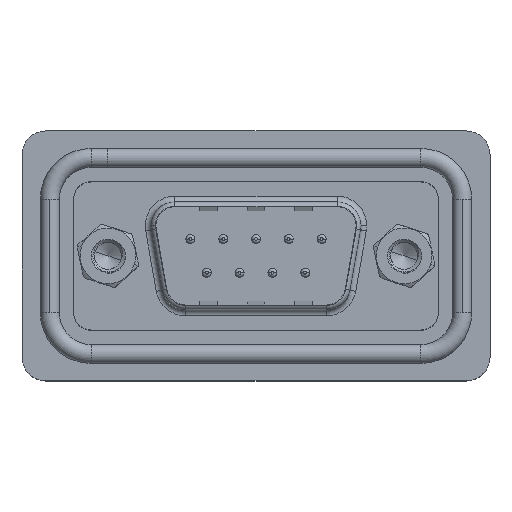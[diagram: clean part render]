
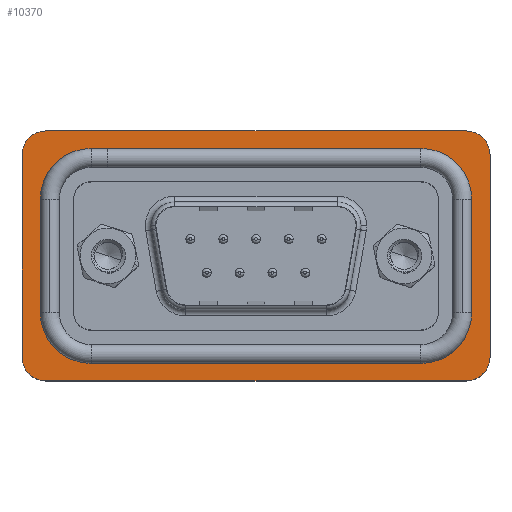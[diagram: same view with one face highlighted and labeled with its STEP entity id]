
A CAD part, top view. The second image highlights one B-rep face of the part: STEP entity #10370.
In plain terms, the highlighted planar face has unit normal (0, 0, 1).
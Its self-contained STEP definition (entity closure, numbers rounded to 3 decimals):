
#96 = LINE ( 'NONE', #14148, #6378 ) ;
#99 = DIRECTION ( 'NONE',  ( 0., 0., 1. ) ) ;
#540 = CIRCLE ( 'NONE', #13585, 4.3 ) ;
#606 = EDGE_CURVE ( 'NONE', #3414, #6151, #19658, .T. ) ;
#797 = CARTESIAN_POINT ( 'NONE',  ( 30.705, -4.775, 0.5 ) ) ;
#854 = VERTEX_POINT ( 'NONE', #5280 ) ;
#891 = CARTESIAN_POINT ( 'NONE',  ( 26.405, 9.075, 0.5 ) ) ;
#929 = VECTOR ( 'NONE', #9782, 1000. ) ;
#997 = CARTESIAN_POINT ( 'NONE',  ( 26.405, 4.775, 0.5 ) ) ;
#1078 = ORIENTED_EDGE ( 'NONE', *, *, #3339, .F. ) ;
#1106 = CARTESIAN_POINT ( 'NONE',  ( -7.25, -8.55, 0.5 ) ) ;
#1278 = VECTOR ( 'NONE', #11512, 1000. ) ;
#1297 = ORIENTED_EDGE ( 'NONE', *, *, #1497, .T. ) ;
#1317 = VERTEX_POINT ( 'NONE', #15199 ) ;
#1422 = ORIENTED_EDGE ( 'NONE', *, *, #11343, .F. ) ;
#1497 = EDGE_CURVE ( 'NONE', #4690, #17657, #9756, .T. ) ;
#1758 = DIRECTION ( 'NONE',  ( 0., 0., 1. ) ) ;
#1893 = VERTEX_POINT ( 'NONE', #797 ) ;
#1958 = DIRECTION ( 'NONE',  ( 1., 0., 0. ) ) ;
#2152 = LINE ( 'NONE', #5312, #1278 ) ;
#2167 = CARTESIAN_POINT ( 'NONE',  ( 30.705, -4.775, 0.5 ) ) ;
#2875 = CARTESIAN_POINT ( 'NONE',  ( 30.25, 8.55, 0.5 ) ) ;
#2889 = DIRECTION ( 'NONE',  ( 0., 0., 1. ) ) ;
#3090 = DIRECTION ( 'NONE',  ( 1., 0., 0. ) ) ;
#3299 = DIRECTION ( 'NONE',  ( 1., 0., 0. ) ) ;
#3339 = EDGE_CURVE ( 'NONE', #8098, #14010, #8241, .T. ) ;
#3414 = VERTEX_POINT ( 'NONE', #17522 ) ;
#3664 = CARTESIAN_POINT ( 'NONE',  ( -7.25, 8.55, 0.5 ) ) ;
#4052 = ORIENTED_EDGE ( 'NONE', *, *, #11380, .F. ) ;
#4205 = CARTESIAN_POINT ( 'NONE',  ( 30.705, 4.775, 0.5 ) ) ;
#4254 = AXIS2_PLACEMENT_3D ( 'NONE', #13463, #19673, #5709 ) ;
#4343 = ORIENTED_EDGE ( 'NONE', *, *, #19286, .T. ) ;
#4385 = ORIENTED_EDGE ( 'NONE', *, *, #15082, .T. ) ;
#4536 = VERTEX_POINT ( 'NONE', #15399 ) ;
#4690 = VERTEX_POINT ( 'NONE', #15882 ) ;
#4802 = VECTOR ( 'NONE', #7313, 1000. ) ;
#4869 = CARTESIAN_POINT ( 'NONE',  ( -5.25, -10.55, 0.5 ) ) ;
#5123 = LINE ( 'NONE', #2167, #19468 ) ;
#5236 = AXIS2_PLACEMENT_3D ( 'NONE', #19566, #7020, #11823 ) ;
#5280 = CARTESIAN_POINT ( 'NONE',  ( 30.25, 10.55, 0.5 ) ) ;
#5312 = CARTESIAN_POINT ( 'NONE',  ( -1.405, -9.075, 0.5 ) ) ;
#5325 = AXIS2_PLACEMENT_3D ( 'NONE', #14061, #99, #1958 ) ;
#5561 = ORIENTED_EDGE ( 'NONE', *, *, #20165, .T. ) ;
#5697 = DIRECTION ( 'NONE',  ( 0., 0., 1. ) ) ;
#5709 = DIRECTION ( 'NONE',  ( 1., 0., 0. ) ) ;
#5882 = AXIS2_PLACEMENT_3D ( 'NONE', #9493, #1758, #3090 ) ;
#5897 = VECTOR ( 'NONE', #3299, 1000. ) ;
#5939 = DIRECTION ( 'NONE',  ( -1., 0., 0. ) ) ;
#6151 = VERTEX_POINT ( 'NONE', #3664 ) ;
#6205 = DIRECTION ( 'NONE',  ( 0., 0., 1. ) ) ;
#6314 = DIRECTION ( 'NONE',  ( 0., 1., 0. ) ) ;
#6378 = VECTOR ( 'NONE', #6314, 1000. ) ;
#6390 = EDGE_CURVE ( 'NONE', #16327, #7993, #9828, .T. ) ;
#6750 = ORIENTED_EDGE ( 'NONE', *, *, #12729, .T. ) ;
#7020 = DIRECTION ( 'NONE',  ( 0., 0., 1. ) ) ;
#7208 = DIRECTION ( 'NONE',  ( 1., 0., 0. ) ) ;
#7313 = DIRECTION ( 'NONE',  ( 0., -1., 0. ) ) ;
#7444 = PLANE ( 'NONE',  #19441 ) ;
#7993 = VERTEX_POINT ( 'NONE', #10981 ) ;
#8098 = VERTEX_POINT ( 'NONE', #18004 ) ;
#8110 = EDGE_CURVE ( 'NONE', #1317, #8098, #17588, .T. ) ;
#8124 = DIRECTION ( 'NONE',  ( 1., 0., 0. ) ) ;
#8241 = CIRCLE ( 'NONE', #5325, 4.3 ) ;
#8303 = CIRCLE ( 'NONE', #10910, 2. ) ;
#8442 = ORIENTED_EDGE ( 'NONE', *, *, #12794, .F. ) ;
#8841 = LINE ( 'NONE', #13536, #17187 ) ;
#8902 = EDGE_LOOP ( 'NONE', ( #4052, #18088, #14301, #8442, #16794, #1422, #1078, #11259 ) ) ;
#8923 = AXIS2_PLACEMENT_3D ( 'NONE', #18648, #6205, #8124 ) ;
#8973 = FACE_OUTER_BOUND ( 'NONE', #13426, .T. ) ;
#8990 = CARTESIAN_POINT ( 'NONE',  ( -5.705, 4.775, 0.5 ) ) ;
#9073 = DIRECTION ( 'NONE',  ( 1., 0., 0. ) ) ;
#9283 = CARTESIAN_POINT ( 'NONE',  ( -5.25, -8.55, 0.5 ) ) ;
#9493 = CARTESIAN_POINT ( 'NONE',  ( 30.25, -8.55, 0.5 ) ) ;
#9601 = DIRECTION ( 'NONE',  ( 0., 1., 0. ) ) ;
#9606 = CARTESIAN_POINT ( 'NONE',  ( -5.705, -4.775, 0.5 ) ) ;
#9682 = CARTESIAN_POINT ( 'NONE',  ( 30.25, 10.55, 0.5 ) ) ;
#9756 = CIRCLE ( 'NONE', #5882, 2. ) ;
#9774 = VERTEX_POINT ( 'NONE', #4869 ) ;
#9782 = DIRECTION ( 'NONE',  ( -1., 0., 0. ) ) ;
#9828 = CIRCLE ( 'NONE', #16680, 4.3 ) ;
#9946 = DIRECTION ( 'NONE',  ( -1., 0., 0. ) ) ;
#10351 = LINE ( 'NONE', #1106, #4802 ) ;
#10370 = ADVANCED_FACE ( 'NONE', ( #15583, #8973 ), #7444, .T. ) ;
#10432 = VECTOR ( 'NONE', #9946, 1000. ) ;
#10876 = VERTEX_POINT ( 'NONE', #14782 ) ;
#10910 = AXIS2_PLACEMENT_3D ( 'NONE', #9283, #2889, #5939 ) ;
#10981 = CARTESIAN_POINT ( 'NONE',  ( -1.405, -9.075, 0.5 ) ) ;
#11259 = ORIENTED_EDGE ( 'NONE', *, *, #8110, .F. ) ;
#11343 = EDGE_CURVE ( 'NONE', #14010, #16327, #8841, .T. ) ;
#11380 = EDGE_CURVE ( 'NONE', #16590, #1317, #540, .T. ) ;
#11383 = EDGE_CURVE ( 'NONE', #6151, #4536, #10351, .T. ) ;
#11512 = DIRECTION ( 'NONE',  ( 1., 0., 0. ) ) ;
#11823 = DIRECTION ( 'NONE',  ( 1., 0., 0. ) ) ;
#11830 = CARTESIAN_POINT ( 'NONE',  ( 32.25, -8.55, 0.5 ) ) ;
#11968 = ORIENTED_EDGE ( 'NONE', *, *, #606, .T. ) ;
#11974 = ORIENTED_EDGE ( 'NONE', *, *, #17279, .T. ) ;
#12003 = DIRECTION ( 'NONE',  ( 0., -1., 0. ) ) ;
#12668 = CARTESIAN_POINT ( 'NONE',  ( 30.25, -10.55, 0.5 ) ) ;
#12729 = EDGE_CURVE ( 'NONE', #854, #3414, #12853, .T. ) ;
#12794 = EDGE_CURVE ( 'NONE', #7993, #10876, #2152, .T. ) ;
#12853 = LINE ( 'NONE', #9682, #929 ) ;
#12856 = EDGE_CURVE ( 'NONE', #1893, #16590, #5123, .T. ) ;
#13426 = EDGE_LOOP ( 'NONE', ( #4385, #6750, #11968, #14557, #4343, #11974, #1297, #5561 ) ) ;
#13463 = CARTESIAN_POINT ( 'NONE',  ( 26.405, -4.775, 0.5 ) ) ;
#13536 = CARTESIAN_POINT ( 'NONE',  ( -5.705, 4.775, 0.5 ) ) ;
#13549 = CARTESIAN_POINT ( 'NONE',  ( -1.405, -4.775, 0.5 ) ) ;
#13585 = AXIS2_PLACEMENT_3D ( 'NONE', #997, #15048, #7208 ) ;
#14010 = VERTEX_POINT ( 'NONE', #8990 ) ;
#14061 = CARTESIAN_POINT ( 'NONE',  ( -1.405, 4.775, 0.5 ) ) ;
#14148 = CARTESIAN_POINT ( 'NONE',  ( 32.25, -8.55, 0.5 ) ) ;
#14301 = ORIENTED_EDGE ( 'NONE', *, *, #14434, .F. ) ;
#14434 = EDGE_CURVE ( 'NONE', #10876, #1893, #15945, .T. ) ;
#14557 = ORIENTED_EDGE ( 'NONE', *, *, #11383, .T. ) ;
#14782 = CARTESIAN_POINT ( 'NONE',  ( 26.405, -9.075, 0.5 ) ) ;
#15048 = DIRECTION ( 'NONE',  ( 0., 0., 1. ) ) ;
#15082 = EDGE_CURVE ( 'NONE', #19301, #854, #18580, .T. ) ;
#15199 = CARTESIAN_POINT ( 'NONE',  ( 26.405, 9.075, 0.5 ) ) ;
#15399 = CARTESIAN_POINT ( 'NONE',  ( -7.25, -8.55, 0.5 ) ) ;
#15583 = FACE_BOUND ( 'NONE', #8902, .T. ) ;
#15882 = CARTESIAN_POINT ( 'NONE',  ( 30.25, -10.55, 0.5 ) ) ;
#15945 = CIRCLE ( 'NONE', #4254, 4.3 ) ;
#16327 = VERTEX_POINT ( 'NONE', #9606 ) ;
#16590 = VERTEX_POINT ( 'NONE', #4205 ) ;
#16680 = AXIS2_PLACEMENT_3D ( 'NONE', #13549, #5697, #19764 ) ;
#16794 = ORIENTED_EDGE ( 'NONE', *, *, #6390, .F. ) ;
#17187 = VECTOR ( 'NONE', #12003, 1000. ) ;
#17235 = LINE ( 'NONE', #12668, #5897 ) ;
#17279 = EDGE_CURVE ( 'NONE', #9774, #4690, #17235, .T. ) ;
#17522 = CARTESIAN_POINT ( 'NONE',  ( -5.25, 10.55, 0.5 ) ) ;
#17588 = LINE ( 'NONE', #891, #10432 ) ;
#17657 = VERTEX_POINT ( 'NONE', #11830 ) ;
#18004 = CARTESIAN_POINT ( 'NONE',  ( -1.405, 9.075, 0.5 ) ) ;
#18088 = ORIENTED_EDGE ( 'NONE', *, *, #12856, .F. ) ;
#18580 = CIRCLE ( 'NONE', #5236, 2. ) ;
#18648 = CARTESIAN_POINT ( 'NONE',  ( -5.25, 8.55, 0.5 ) ) ;
#19286 = EDGE_CURVE ( 'NONE', #4536, #9774, #8303, .T. ) ;
#19301 = VERTEX_POINT ( 'NONE', #19797 ) ;
#19441 = AXIS2_PLACEMENT_3D ( 'NONE', #2875, #19890, #9073 ) ;
#19468 = VECTOR ( 'NONE', #9601, 1000. ) ;
#19566 = CARTESIAN_POINT ( 'NONE',  ( 30.25, 8.55, 0.5 ) ) ;
#19658 = CIRCLE ( 'NONE', #8923, 2. ) ;
#19673 = DIRECTION ( 'NONE',  ( 0., 0., 1. ) ) ;
#19764 = DIRECTION ( 'NONE',  ( 1., 0., 0. ) ) ;
#19797 = CARTESIAN_POINT ( 'NONE',  ( 32.25, 8.55, 0.5 ) ) ;
#19890 = DIRECTION ( 'NONE',  ( 0., 0., 1. ) ) ;
#20165 = EDGE_CURVE ( 'NONE', #17657, #19301, #96, .T. ) ;
